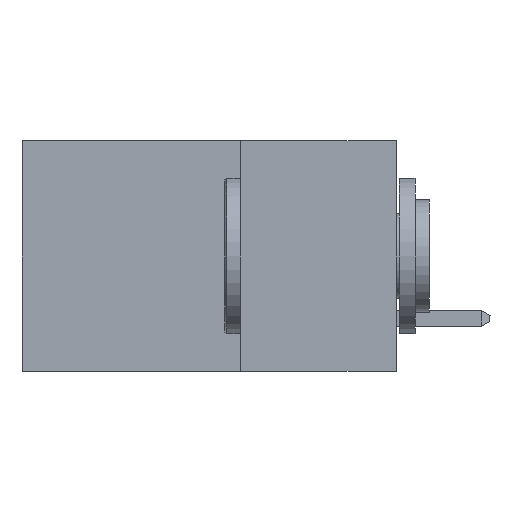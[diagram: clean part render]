
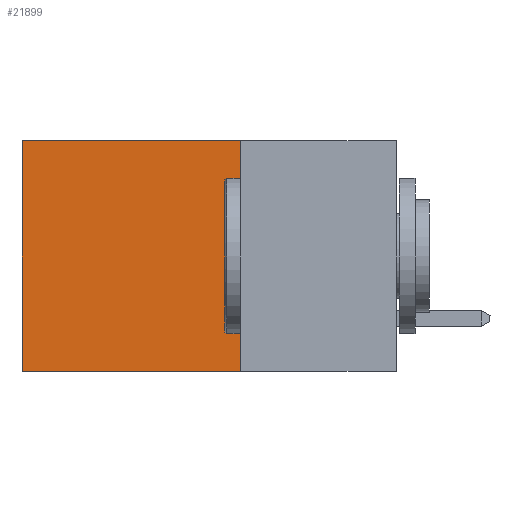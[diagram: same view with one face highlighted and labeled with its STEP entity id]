
A CAD part, left-side view. The second image highlights one B-rep face of the part: STEP entity #21899.
In plain terms, the highlighted planar face has unit normal (-1, 0, 0).
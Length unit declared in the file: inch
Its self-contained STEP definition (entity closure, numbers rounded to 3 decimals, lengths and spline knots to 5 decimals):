
#1069 = LINE ( 'NONE', #4746, #5528 ) ;
#1367 = EDGE_CURVE ( 'NONE', #13339, #10470, #21231, .T. ) ;
#2274 = EDGE_LOOP ( 'NONE', ( #8194, #3368, #6133, #5398 ) ) ;
#2880 = VECTOR ( 'NONE', #5690, 39.37008 ) ;
#3108 = EDGE_CURVE ( 'NONE', #19310, #13339, #1069, .T. ) ;
#3368 = ORIENTED_EDGE ( 'NONE', *, *, #5036, .F. ) ;
#3652 = AXIS2_PLACEMENT_3D ( 'NONE', #15205, #4122, #17052 ) ;
#4122 = DIRECTION ( 'NONE',  ( 1., 0., 0. ) ) ;
#4586 = VECTOR ( 'NONE', #6592, 39.37008 ) ;
#4746 = CARTESIAN_POINT ( 'NONE',  ( 0.2615, 0.25, 0. ) ) ;
#4832 = CARTESIAN_POINT ( 'NONE',  ( 0.2615, 0.6, -0.37 ) ) ;
#4842 = CARTESIAN_POINT ( 'NONE',  ( 0.2615, 0.25, -0.37 ) ) ;
#4875 = DIRECTION ( 'NONE',  ( 0., 1., 0. ) ) ;
#5036 = EDGE_CURVE ( 'NONE', #16334, #10470, #18703, .T. ) ;
#5398 = ORIENTED_EDGE ( 'NONE', *, *, #3108, .T. ) ;
#5528 = VECTOR ( 'NONE', #4875, 39.37008 ) ;
#5680 = CARTESIAN_POINT ( 'NONE',  ( 0.2615, 0.6, -0.37 ) ) ;
#5690 = DIRECTION ( 'NONE',  ( 0., 0., -1. ) ) ;
#6064 = EDGE_CURVE ( 'NONE', #19310, #16334, #17671, .T. ) ;
#6133 = ORIENTED_EDGE ( 'NONE', *, *, #6064, .F. ) ;
#6206 = CARTESIAN_POINT ( 'NONE',  ( 0.2615, 0.25, -0.37 ) ) ;
#6592 = DIRECTION ( 'NONE',  ( 0., 1., 0. ) ) ;
#6817 = VECTOR ( 'NONE', #7497, 39.37008 ) ;
#7497 = DIRECTION ( 'NONE',  ( 0., 0., -1. ) ) ;
#8194 = ORIENTED_EDGE ( 'NONE', *, *, #1367, .T. ) ;
#8925 = CARTESIAN_POINT ( 'NONE',  ( 0.2615, 0.6, 0. ) ) ;
#10470 = VERTEX_POINT ( 'NONE', #4832 ) ;
#11579 = PLANE ( 'NONE',  #3652 ) ;
#13339 = VERTEX_POINT ( 'NONE', #8925 ) ;
#15205 = CARTESIAN_POINT ( 'NONE',  ( 0.2615, 0.25, -0.37 ) ) ;
#15569 = CARTESIAN_POINT ( 'NONE',  ( 0.2615, 0.25, -0.37 ) ) ;
#16334 = VERTEX_POINT ( 'NONE', #15569 ) ;
#17052 = DIRECTION ( 'NONE',  ( 0., 0., -1. ) ) ;
#17671 = LINE ( 'NONE', #4842, #2880 ) ;
#18703 = LINE ( 'NONE', #6206, #4586 ) ;
#19310 = VERTEX_POINT ( 'NONE', #22934 ) ;
#21231 = LINE ( 'NONE', #5680, #6817 ) ;
#21899 = ADVANCED_FACE ( 'NONE', ( #23265 ), #11579, .F. ) ;
#22934 = CARTESIAN_POINT ( 'NONE',  ( 0.2615, 0.25, 0. ) ) ;
#23265 = FACE_OUTER_BOUND ( 'NONE', #2274, .T. ) ;
